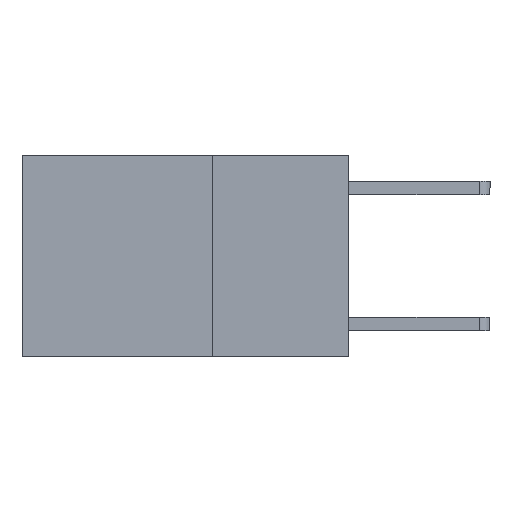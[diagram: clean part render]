
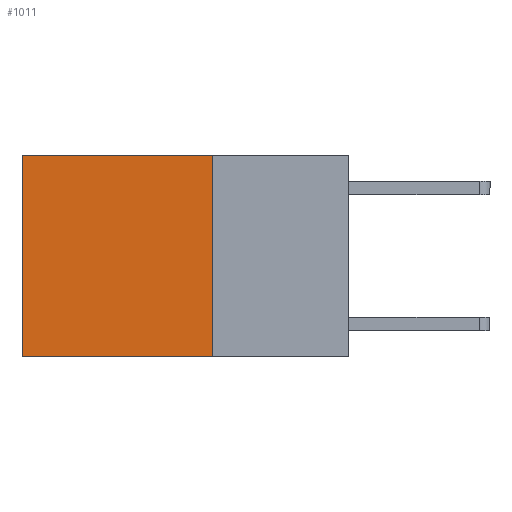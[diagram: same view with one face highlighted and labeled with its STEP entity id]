
A CAD part, left-side view. The second image highlights one B-rep face of the part: STEP entity #1011.
In plain terms, the highlighted planar face has unit normal (-1, 0, 0).
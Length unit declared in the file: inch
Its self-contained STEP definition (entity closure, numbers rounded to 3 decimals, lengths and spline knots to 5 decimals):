
#32 = DIRECTION ( 'NONE',  ( 0., 1., 0. ) ) ;
#256 = DIRECTION ( 'NONE',  ( 1., 0., 0. ) ) ;
#349 = EDGE_CURVE ( 'NONE', #550, #6161, #5745, .T. ) ;
#550 = VERTEX_POINT ( 'NONE', #5872 ) ;
#1011 = ADVANCED_FACE ( 'NONE', ( #2531 ), #8113, .F. ) ;
#1343 = ORIENTED_EDGE ( 'NONE', *, *, #5272, .T. ) ;
#1978 = DIRECTION ( 'NONE',  ( 0., 0., -1. ) ) ;
#2531 = FACE_OUTER_BOUND ( 'NONE', #6624, .T. ) ;
#2745 = VERTEX_POINT ( 'NONE', #4597 ) ;
#3129 = DIRECTION ( 'NONE',  ( 0., 0., -1. ) ) ;
#3179 = VECTOR ( 'NONE', #3332, 39.37008 ) ;
#3270 = VECTOR ( 'NONE', #32, 39.37008 ) ;
#3332 = DIRECTION ( 'NONE',  ( 0., 0., -1. ) ) ;
#3595 = LINE ( 'NONE', #5129, #4682 ) ;
#4039 = VERTEX_POINT ( 'NONE', #5910 ) ;
#4277 = VECTOR ( 'NONE', #1978, 39.37008 ) ;
#4597 = CARTESIAN_POINT ( 'NONE',  ( 0.2625, 0.25, 0. ) ) ;
#4682 = VECTOR ( 'NONE', #6438, 39.37008 ) ;
#4724 = EDGE_CURVE ( 'NONE', #2745, #550, #7674, .T. ) ;
#4737 = AXIS2_PLACEMENT_3D ( 'NONE', #6659, #256, #3129 ) ;
#5129 = CARTESIAN_POINT ( 'NONE',  ( 0.2625, 0.25, 0. ) ) ;
#5272 = EDGE_CURVE ( 'NONE', #2745, #4039, #3595, .T. ) ;
#5745 = LINE ( 'NONE', #6386, #3270 ) ;
#5872 = CARTESIAN_POINT ( 'NONE',  ( 0.2625, 0.25, -0.37 ) ) ;
#5910 = CARTESIAN_POINT ( 'NONE',  ( 0.2625, 0.6, 0. ) ) ;
#6133 = LINE ( 'NONE', #6890, #4277 ) ;
#6161 = VERTEX_POINT ( 'NONE', #6511 ) ;
#6386 = CARTESIAN_POINT ( 'NONE',  ( 0.2625, 0.25, -0.37 ) ) ;
#6416 = ORIENTED_EDGE ( 'NONE', *, *, #349, .F. ) ;
#6428 = ORIENTED_EDGE ( 'NONE', *, *, #4724, .F. ) ;
#6438 = DIRECTION ( 'NONE',  ( 0., 1., 0. ) ) ;
#6511 = CARTESIAN_POINT ( 'NONE',  ( 0.2625, 0.6, -0.37 ) ) ;
#6624 = EDGE_LOOP ( 'NONE', ( #8433, #6416, #6428, #1343 ) ) ;
#6659 = CARTESIAN_POINT ( 'NONE',  ( 0.2625, 0.25, 0. ) ) ;
#6890 = CARTESIAN_POINT ( 'NONE',  ( 0.2625, 0.6, 0. ) ) ;
#7644 = EDGE_CURVE ( 'NONE', #4039, #6161, #6133, .T. ) ;
#7674 = LINE ( 'NONE', #8184, #3179 ) ;
#8113 = PLANE ( 'NONE',  #4737 ) ;
#8184 = CARTESIAN_POINT ( 'NONE',  ( 0.2625, 0.25, 0. ) ) ;
#8433 = ORIENTED_EDGE ( 'NONE', *, *, #7644, .T. ) ;
